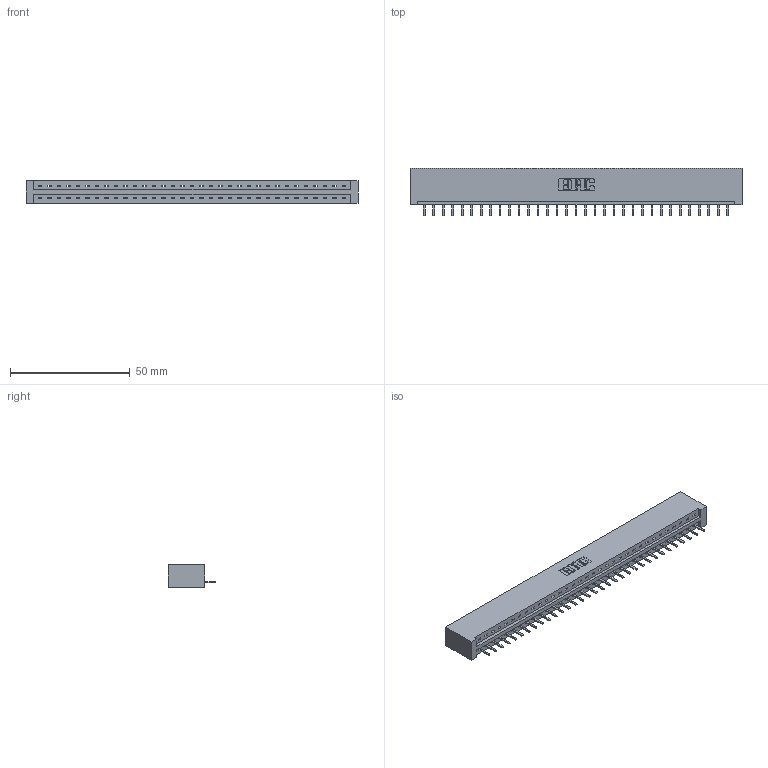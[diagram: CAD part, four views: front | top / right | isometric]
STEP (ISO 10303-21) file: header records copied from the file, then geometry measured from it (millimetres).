
FILE_DESCRIPTION (( 'STEP AP203' ), '1' );
FILE_NAME ('337-033-520-101.STEP', '2018-08-07T08:02:34', ( '' ), ( '' ), 'SwSTEP 2.0', 'SolidWorks 2016', '' );
FILE_SCHEMA (( 'CONFIG_CONTROL_DESIGN' ));
Length unit declared in the file: inch
Products named in the file (3): 337 Part_No Mounting Lugs; 345-292-001_345-293-120; 337-033-520-101
Assembly tree (34 placements, depth 2):
  337-033-520-101
    337 Part_No Mounting Lugs
    345-292-001_345-293-120  x33
Bounding box: 138.63 x 20.02 x 9.4 mm (x, y, z)
Volume: 14939.8 mm3; surface area: 15027.8 mm2
Topology: 34 solids, 34 shells, 2284 faces, 6755 edges, 4414 vertices
Faces by surface type: plane 1650, cylinder 634
Entity records: 25531 total; most frequent: CARTESIAN_POINT 4465, ORIENTED_EDGE 4422, DIRECTION 3757, EDGE_CURVE 2211, VECTOR 2087, LINE 2087, VERTEX_POINT 1470, AXIS2_PLACEMENT_3D 835
